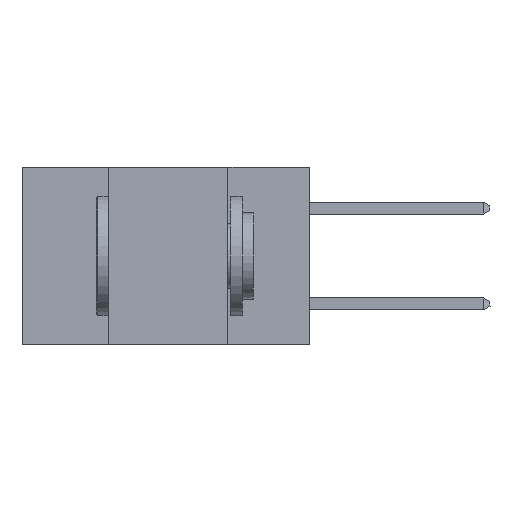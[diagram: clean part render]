
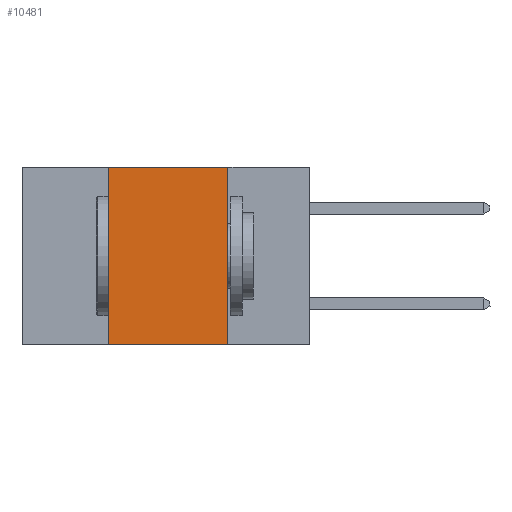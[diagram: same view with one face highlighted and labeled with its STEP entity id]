
A CAD part, left-side view. The second image highlights one B-rep face of the part: STEP entity #10481.
In plain terms, the highlighted planar face has unit normal (-1, 0, 0).
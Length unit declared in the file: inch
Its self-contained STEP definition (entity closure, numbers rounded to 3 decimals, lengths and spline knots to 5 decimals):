
#558 = ORIENTED_EDGE ( 'NONE', *, *, #11947, .F. ) ;
#860 = EDGE_LOOP ( 'NONE', ( #558, #11559, #15316, #10746 ) ) ;
#1705 = VERTEX_POINT ( 'NONE', #18675 ) ;
#2141 = LINE ( 'NONE', #22243, #20105 ) ;
#2556 = AXIS2_PLACEMENT_3D ( 'NONE', #18704, #3133, #15365 ) ;
#3133 = DIRECTION ( 'NONE',  ( 1., 0., 0. ) ) ;
#5030 = LINE ( 'NONE', #16716, #18323 ) ;
#5130 = VERTEX_POINT ( 'NONE', #11223 ) ;
#5762 = CARTESIAN_POINT ( 'NONE',  ( 0., 0.17, 0. ) ) ;
#5857 = CARTESIAN_POINT ( 'NONE',  ( 0., 0.42, 0. ) ) ;
#5858 = FACE_OUTER_BOUND ( 'NONE', #860, .T. ) ;
#6055 = CARTESIAN_POINT ( 'NONE',  ( 0., 0.17, 0. ) ) ;
#7638 = DIRECTION ( 'NONE',  ( 0., 0., 1. ) ) ;
#7887 = VERTEX_POINT ( 'NONE', #5762 ) ;
#8540 = VECTOR ( 'NONE', #18261, 39.37008 ) ;
#10481 = ADVANCED_FACE ( 'NONE', ( #5858 ), #11853, .F. ) ;
#10746 = ORIENTED_EDGE ( 'NONE', *, *, #19518, .T. ) ;
#11223 = CARTESIAN_POINT ( 'NONE',  ( 0., 0.42, 0. ) ) ;
#11559 = ORIENTED_EDGE ( 'NONE', *, *, #16225, .F. ) ;
#11853 = PLANE ( 'NONE',  #2556 ) ;
#11940 = DIRECTION ( 'NONE',  ( 0., -1., 0. ) ) ;
#11947 = EDGE_CURVE ( 'NONE', #7887, #1705, #17696, .T. ) ;
#12962 = VERTEX_POINT ( 'NONE', #17462 ) ;
#13598 = VECTOR ( 'NONE', #7638, 39.37008 ) ;
#15316 = ORIENTED_EDGE ( 'NONE', *, *, #21551, .F. ) ;
#15365 = DIRECTION ( 'NONE',  ( 0., 0., -1. ) ) ;
#16225 = EDGE_CURVE ( 'NONE', #5130, #7887, #5030, .T. ) ;
#16716 = CARTESIAN_POINT ( 'NONE',  ( 0., 0.6, 0. ) ) ;
#17462 = CARTESIAN_POINT ( 'NONE',  ( 0., 0.42, -0.37 ) ) ;
#17696 = LINE ( 'NONE', #6055, #8540 ) ;
#18261 = DIRECTION ( 'NONE',  ( 0., 0., -1. ) ) ;
#18323 = VECTOR ( 'NONE', #18435, 39.37008 ) ;
#18435 = DIRECTION ( 'NONE',  ( 0., -1., 0. ) ) ;
#18675 = CARTESIAN_POINT ( 'NONE',  ( 0., 0.17, -0.37 ) ) ;
#18704 = CARTESIAN_POINT ( 'NONE',  ( 0., 0.6, 0. ) ) ;
#19186 = LINE ( 'NONE', #5857, #13598 ) ;
#19518 = EDGE_CURVE ( 'NONE', #12962, #1705, #2141, .T. ) ;
#20105 = VECTOR ( 'NONE', #11940, 39.37008 ) ;
#21551 = EDGE_CURVE ( 'NONE', #12962, #5130, #19186, .T. ) ;
#22243 = CARTESIAN_POINT ( 'NONE',  ( 0., 0.6, -0.37 ) ) ;
